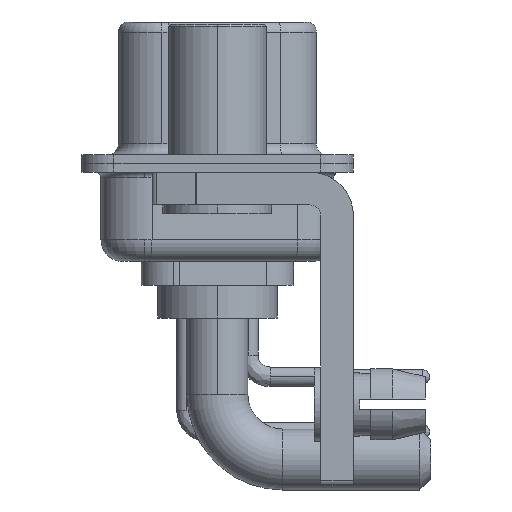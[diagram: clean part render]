
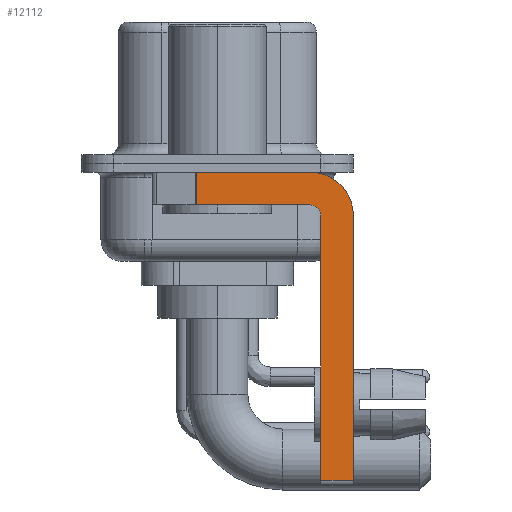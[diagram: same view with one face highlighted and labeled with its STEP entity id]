
A CAD part, left-side view. The second image highlights one B-rep face of the part: STEP entity #12112.
In plain terms, the highlighted planar face has unit normal (-1, 0, 0).
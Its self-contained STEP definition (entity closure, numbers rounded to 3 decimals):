
#28 = CIRCLE ( 'NONE', #21103, 0.5 ) ;
#356 = EDGE_CURVE ( 'NONE', #6165, #4655, #28, .T. ) ;
#431 = LINE ( 'NONE', #14121, #9195 ) ;
#585 = DIRECTION ( 'NONE',  ( -1., 0., 0. ) ) ;
#2066 = CARTESIAN_POINT ( 'NONE',  ( -2.9, 0.978, -0.4 ) ) ;
#2429 = EDGE_CURVE ( 'NONE', #4617, #18085, #6000, .T. ) ;
#2989 = VECTOR ( 'NONE', #20761, 1000. ) ;
#3085 = LINE ( 'NONE', #8662, #15520 ) ;
#3261 = LINE ( 'NONE', #9461, #2989 ) ;
#3940 = EDGE_CURVE ( 'NONE', #4088, #18085, #3085, .T. ) ;
#4088 = VERTEX_POINT ( 'NONE', #15639 ) ;
#4102 = ORIENTED_EDGE ( 'NONE', *, *, #19573, .F. ) ;
#4161 = CARTESIAN_POINT ( 'NONE',  ( -2.9, -4.25, -2.4 ) ) ;
#4617 = VERTEX_POINT ( 'NONE', #23198 ) ;
#4655 = VERTEX_POINT ( 'NONE', #9757 ) ;
#4891 = ORIENTED_EDGE ( 'NONE', *, *, #7853, .F. ) ;
#5133 = VECTOR ( 'NONE', #24768, 1000. ) ;
#5139 = ORIENTED_EDGE ( 'NONE', *, *, #3940, .F. ) ;
#6000 = LINE ( 'NONE', #13732, #5133 ) ;
#6165 = VERTEX_POINT ( 'NONE', #16995 ) ;
#6401 = VECTOR ( 'NONE', #23854, 1000. ) ;
#6588 = LINE ( 'NONE', #13827, #6401 ) ;
#6708 = CARTESIAN_POINT ( 'NONE',  ( -2.9, -4.25, -1.9 ) ) ;
#6739 = AXIS2_PLACEMENT_3D ( 'NONE', #4161, #10130, #18240 ) ;
#7853 = EDGE_CURVE ( 'NONE', #14852, #24515, #3261, .T. ) ;
#8648 = DIRECTION ( 'NONE',  ( 1., 0., 0. ) ) ;
#8662 = CARTESIAN_POINT ( 'NONE',  ( -2.9, -6.25, -2.4 ) ) ;
#8904 = DIRECTION ( 'NONE',  ( 0., 0., -1. ) ) ;
#9195 = VECTOR ( 'NONE', #10562, 1000. ) ;
#9461 = CARTESIAN_POINT ( 'NONE',  ( -2.9, 3., -0.4 ) ) ;
#9757 = CARTESIAN_POINT ( 'NONE',  ( -2.9, -4.25, -1.9 ) ) ;
#10130 = DIRECTION ( 'NONE',  ( 1., 0., 0. ) ) ;
#10437 = CARTESIAN_POINT ( 'NONE',  ( -2.9, 0.978, -1.9 ) ) ;
#10562 = DIRECTION ( 'NONE',  ( 0., 0., 1. ) ) ;
#10667 = FACE_OUTER_BOUND ( 'NONE', #15643, .T. ) ;
#10880 = DIRECTION ( 'NONE',  ( 0., 1., 0. ) ) ;
#11672 = ORIENTED_EDGE ( 'NONE', *, *, #13570, .T. ) ;
#11880 = ORIENTED_EDGE ( 'NONE', *, *, #356, .F. ) ;
#12112 = ADVANCED_FACE ( 'NONE', ( #10667 ), #18174, .F. ) ;
#12851 = AXIS2_PLACEMENT_3D ( 'NONE', #22338, #8648, #8904 ) ;
#13570 = EDGE_CURVE ( 'NONE', #14852, #14430, #6588, .T. ) ;
#13732 = CARTESIAN_POINT ( 'NONE',  ( -2.9, -4.25, -14.55 ) ) ;
#13827 = CARTESIAN_POINT ( 'NONE',  ( -2.9, 0.978, -1.9 ) ) ;
#13897 = VECTOR ( 'NONE', #10880, 1000. ) ;
#14020 = DIRECTION ( 'NONE',  ( 0., 0., 1. ) ) ;
#14121 = CARTESIAN_POINT ( 'NONE',  ( -2.9, -4.75, -14.8 ) ) ;
#14430 = VERTEX_POINT ( 'NONE', #10437 ) ;
#14478 = ORIENTED_EDGE ( 'NONE', *, *, #22259, .F. ) ;
#14852 = VERTEX_POINT ( 'NONE', #2066 ) ;
#15520 = VECTOR ( 'NONE', #16908, 1000. ) ;
#15639 = CARTESIAN_POINT ( 'NONE',  ( -2.9, -6.25, -2.4 ) ) ;
#15643 = EDGE_LOOP ( 'NONE', ( #4891, #11672, #4102, #11880, #17864, #17842, #5139, #14478 ) ) ;
#16046 = CARTESIAN_POINT ( 'NONE',  ( -2.9, -4.25, -0.4 ) ) ;
#16056 = CIRCLE ( 'NONE', #6739, 2. ) ;
#16864 = LINE ( 'NONE', #6708, #13897 ) ;
#16908 = DIRECTION ( 'NONE',  ( 0., 0., -1. ) ) ;
#16995 = CARTESIAN_POINT ( 'NONE',  ( -2.9, -4.75, -2.4 ) ) ;
#17842 = ORIENTED_EDGE ( 'NONE', *, *, #2429, .T. ) ;
#17864 = ORIENTED_EDGE ( 'NONE', *, *, #24472, .F. ) ;
#18085 = VERTEX_POINT ( 'NONE', #19540 ) ;
#18174 = PLANE ( 'NONE',  #12851 ) ;
#18240 = DIRECTION ( 'NONE',  ( 0., 0., -1. ) ) ;
#19540 = CARTESIAN_POINT ( 'NONE',  ( -2.9, -6.25, -14.55 ) ) ;
#19573 = EDGE_CURVE ( 'NONE', #4655, #14430, #16864, .T. ) ;
#20761 = DIRECTION ( 'NONE',  ( 0., -1., 0. ) ) ;
#21103 = AXIS2_PLACEMENT_3D ( 'NONE', #21528, #585, #14020 ) ;
#21528 = CARTESIAN_POINT ( 'NONE',  ( -2.9, -4.25, -2.4 ) ) ;
#22259 = EDGE_CURVE ( 'NONE', #24515, #4088, #16056, .T. ) ;
#22338 = CARTESIAN_POINT ( 'NONE',  ( -2.9, -4.25, -2.4 ) ) ;
#23198 = CARTESIAN_POINT ( 'NONE',  ( -2.9, -4.75, -14.55 ) ) ;
#23854 = DIRECTION ( 'NONE',  ( 0., 0., -1. ) ) ;
#24472 = EDGE_CURVE ( 'NONE', #4617, #6165, #431, .T. ) ;
#24515 = VERTEX_POINT ( 'NONE', #16046 ) ;
#24768 = DIRECTION ( 'NONE',  ( 0., -1., 0. ) ) ;
